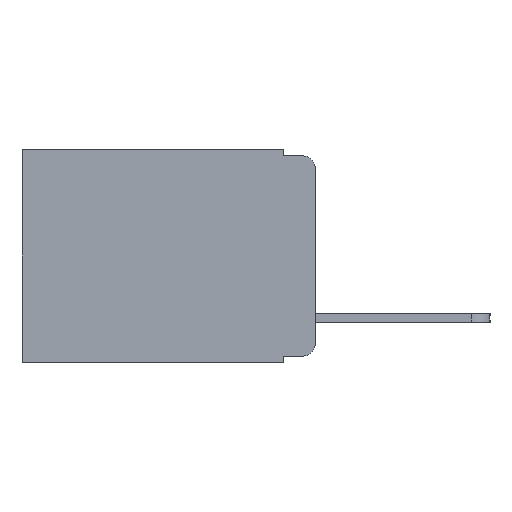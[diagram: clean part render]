
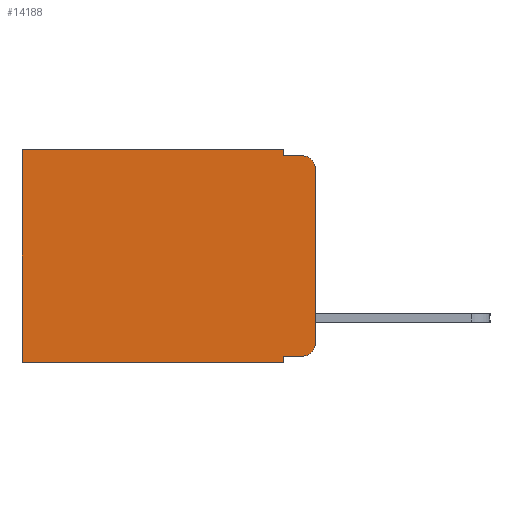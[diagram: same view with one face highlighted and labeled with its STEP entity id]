
A CAD part, left-side view. The second image highlights one B-rep face of the part: STEP entity #14188.
In plain terms, the highlighted planar face has unit normal (-1, 0, 0).
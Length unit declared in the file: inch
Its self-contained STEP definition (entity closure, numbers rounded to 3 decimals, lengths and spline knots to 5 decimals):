
#76 = LINE ( 'NONE', #6894, #12585 ) ;
#250 = LINE ( 'NONE', #6943, #15271 ) ;
#258 = ORIENTED_EDGE ( 'NONE', *, *, #15001, .T. ) ;
#791 = LINE ( 'NONE', #15395, #13461 ) ;
#814 = VERTEX_POINT ( 'NONE', #5921 ) ;
#858 = ORIENTED_EDGE ( 'NONE', *, *, #7422, .T. ) ;
#890 = ORIENTED_EDGE ( 'NONE', *, *, #14449, .F. ) ;
#919 = EDGE_CURVE ( 'NONE', #5338, #814, #7829, .T. ) ;
#964 = EDGE_LOOP ( 'NONE', ( #1658, #1969, #10818, #12008, #858, #10554, #890, #7013, #6107, #258 ) ) ;
#1038 = VERTEX_POINT ( 'NONE', #9276 ) ;
#1152 = CARTESIAN_POINT ( 'NONE',  ( 0.298, 0.02, -0.01 ) ) ;
#1275 = DIRECTION ( 'NONE',  ( 0., 0., -1. ) ) ;
#1311 = VERTEX_POINT ( 'NONE', #11004 ) ;
#1658 = ORIENTED_EDGE ( 'NONE', *, *, #7809, .F. ) ;
#1822 = EDGE_CURVE ( 'NONE', #1311, #1038, #9331, .T. ) ;
#1969 = ORIENTED_EDGE ( 'NONE', *, *, #5249, .T. ) ;
#2008 = CARTESIAN_POINT ( 'NONE',  ( 0.298, 0., 0. ) ) ;
#2346 = CARTESIAN_POINT ( 'NONE',  ( 0.298, 0.02, -0.03 ) ) ;
#2565 = DIRECTION ( 'NONE',  ( -1., 0., 0. ) ) ;
#2734 = EDGE_CURVE ( 'NONE', #7877, #7054, #250, .T. ) ;
#2875 = CARTESIAN_POINT ( 'NONE',  ( 0.298, 0.473, 0. ) ) ;
#2993 = DIRECTION ( 'NONE',  ( 0., 1., 0. ) ) ;
#3067 = VECTOR ( 'NONE', #14205, 39.37008 ) ;
#3597 = EDGE_CURVE ( 'NONE', #7054, #6708, #5356, .T. ) ;
#4123 = AXIS2_PLACEMENT_3D ( 'NONE', #7326, #13196, #6109 ) ;
#4294 = CARTESIAN_POINT ( 'NONE',  ( 0.298, 0.02, -0.333 ) ) ;
#4486 = VECTOR ( 'NONE', #1275, 39.37008 ) ;
#4894 = DIRECTION ( 'NONE',  ( 0., -1., 0. ) ) ;
#5249 = EDGE_CURVE ( 'NONE', #12943, #6708, #15533, .T. ) ;
#5286 = CARTESIAN_POINT ( 'NONE',  ( 0.298, 0., -0.343 ) ) ;
#5338 = VERTEX_POINT ( 'NONE', #9828 ) ;
#5356 = LINE ( 'NONE', #8098, #14400 ) ;
#5392 = CARTESIAN_POINT ( 'NONE',  ( 0.298, 0., -0.313 ) ) ;
#5921 = CARTESIAN_POINT ( 'NONE',  ( 0.298, 0.051, -0.343 ) ) ;
#6107 = ORIENTED_EDGE ( 'NONE', *, *, #15706, .T. ) ;
#6109 = DIRECTION ( 'NONE',  ( 0., 0., -1. ) ) ;
#6708 = VERTEX_POINT ( 'NONE', #1152 ) ;
#6894 = CARTESIAN_POINT ( 'NONE',  ( 0.298, 0., 0. ) ) ;
#6943 = CARTESIAN_POINT ( 'NONE',  ( 0.298, 0.051, 0. ) ) ;
#7013 = ORIENTED_EDGE ( 'NONE', *, *, #919, .F. ) ;
#7054 = VERTEX_POINT ( 'NONE', #12201 ) ;
#7269 = CARTESIAN_POINT ( 'NONE',  ( 0.298, 0.051, 0. ) ) ;
#7322 = CARTESIAN_POINT ( 'NONE',  ( 0.298, 0.02, -0.313 ) ) ;
#7326 = CARTESIAN_POINT ( 'NONE',  ( 0.298, 0., 0. ) ) ;
#7422 = EDGE_CURVE ( 'NONE', #7877, #1311, #76, .T. ) ;
#7809 = EDGE_CURVE ( 'NONE', #12943, #9421, #10273, .T. ) ;
#7829 = LINE ( 'NONE', #10618, #4486 ) ;
#7877 = VERTEX_POINT ( 'NONE', #7269 ) ;
#8098 = CARTESIAN_POINT ( 'NONE',  ( 0.298, 0.051, -0.01 ) ) ;
#8520 = DIRECTION ( 'NONE',  ( 0., 0., -1. ) ) ;
#8849 = VERTEX_POINT ( 'NONE', #4294 ) ;
#9276 = CARTESIAN_POINT ( 'NONE',  ( 0.298, 0.473, -0.343 ) ) ;
#9312 = CIRCLE ( 'NONE', #13897, 0.02 ) ;
#9331 = LINE ( 'NONE', #2875, #3067 ) ;
#9421 = VERTEX_POINT ( 'NONE', #5392 ) ;
#9766 = PLANE ( 'NONE',  #4123 ) ;
#9828 = CARTESIAN_POINT ( 'NONE',  ( 0.298, 0.051, -0.333 ) ) ;
#10273 = LINE ( 'NONE', #2008, #12930 ) ;
#10554 = ORIENTED_EDGE ( 'NONE', *, *, #1822, .T. ) ;
#10618 = CARTESIAN_POINT ( 'NONE',  ( 0.298, 0.051, 0. ) ) ;
#10818 = ORIENTED_EDGE ( 'NONE', *, *, #3597, .F. ) ;
#11004 = CARTESIAN_POINT ( 'NONE',  ( 0.298, 0.473, 0. ) ) ;
#11142 = AXIS2_PLACEMENT_3D ( 'NONE', #2346, #2565, #11229 ) ;
#11192 = VECTOR ( 'NONE', #13605, 39.37008 ) ;
#11229 = DIRECTION ( 'NONE',  ( 0., 0., -1. ) ) ;
#12008 = ORIENTED_EDGE ( 'NONE', *, *, #2734, .F. ) ;
#12092 = FACE_OUTER_BOUND ( 'NONE', #964, .T. ) ;
#12201 = CARTESIAN_POINT ( 'NONE',  ( 0.298, 0.051, -0.01 ) ) ;
#12585 = VECTOR ( 'NONE', #2993, 39.37008 ) ;
#12930 = VECTOR ( 'NONE', #13010, 39.37008 ) ;
#12943 = VERTEX_POINT ( 'NONE', #13038 ) ;
#13010 = DIRECTION ( 'NONE',  ( 0., 0., -1. ) ) ;
#13038 = CARTESIAN_POINT ( 'NONE',  ( 0.298, 0., -0.03 ) ) ;
#13157 = DIRECTION ( 'NONE',  ( 0., 0., -1. ) ) ;
#13196 = DIRECTION ( 'NONE',  ( 1., 0., 0. ) ) ;
#13461 = VECTOR ( 'NONE', #4894, 39.37008 ) ;
#13605 = DIRECTION ( 'NONE',  ( 0., 1., 0. ) ) ;
#13897 = AXIS2_PLACEMENT_3D ( 'NONE', #7322, #15321, #8520 ) ;
#14118 = LINE ( 'NONE', #5286, #11192 ) ;
#14188 = ADVANCED_FACE ( 'NONE', ( #12092 ), #9766, .F. ) ;
#14205 = DIRECTION ( 'NONE',  ( 0., 0., -1. ) ) ;
#14400 = VECTOR ( 'NONE', #14513, 39.37008 ) ;
#14449 = EDGE_CURVE ( 'NONE', #814, #1038, #14118, .T. ) ;
#14513 = DIRECTION ( 'NONE',  ( 0., -1., 0. ) ) ;
#15001 = EDGE_CURVE ( 'NONE', #8849, #9421, #9312, .T. ) ;
#15271 = VECTOR ( 'NONE', #13157, 39.37008 ) ;
#15321 = DIRECTION ( 'NONE',  ( -1., 0., 0. ) ) ;
#15395 = CARTESIAN_POINT ( 'NONE',  ( 0.298, 0.051, -0.333 ) ) ;
#15533 = CIRCLE ( 'NONE', #11142, 0.02 ) ;
#15706 = EDGE_CURVE ( 'NONE', #5338, #8849, #791, .T. ) ;
